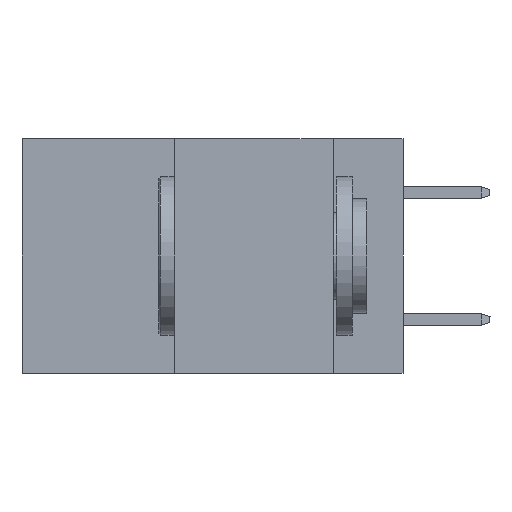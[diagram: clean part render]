
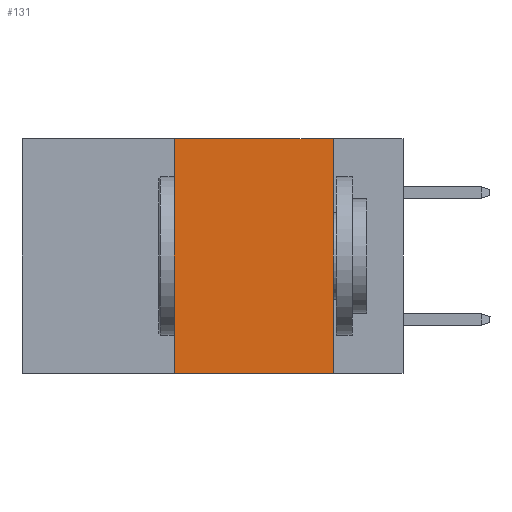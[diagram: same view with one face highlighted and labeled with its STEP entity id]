
A CAD part, left-side view. The second image highlights one B-rep face of the part: STEP entity #131.
In plain terms, the highlighted planar face has unit normal (-1, 0, 0).
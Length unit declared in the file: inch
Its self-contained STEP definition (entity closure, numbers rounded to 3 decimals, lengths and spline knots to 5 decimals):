
#131 = ADVANCED_FACE ( 'NONE', ( #4644 ), #4744, .F. ) ;
#813 = ORIENTED_EDGE ( 'NONE', *, *, #11882, .F. ) ;
#826 = DIRECTION ( 'NONE',  ( 0., -1., 0. ) ) ;
#1549 = LINE ( 'NONE', #8053, #18817 ) ;
#1896 = EDGE_CURVE ( 'NONE', #18761, #7512, #11282, .T. ) ;
#2159 = LINE ( 'NONE', #8363, #12475 ) ;
#2453 = DIRECTION ( 'NONE',  ( 0., 0., 1. ) ) ;
#3088 = ORIENTED_EDGE ( 'NONE', *, *, #19237, .F. ) ;
#3371 = DIRECTION ( 'NONE',  ( 0., 0., -1. ) ) ;
#3776 = ORIENTED_EDGE ( 'NONE', *, *, #13937, .T. ) ;
#4063 = CARTESIAN_POINT ( 'NONE',  ( 0., 0.6, 0. ) ) ;
#4644 = FACE_OUTER_BOUND ( 'NONE', #6862, .T. ) ;
#4744 = PLANE ( 'NONE',  #14690 ) ;
#6140 = CARTESIAN_POINT ( 'NONE',  ( 0., 0.36, -0.37 ) ) ;
#6268 = DIRECTION ( 'NONE',  ( 1., 0., 0. ) ) ;
#6569 = CARTESIAN_POINT ( 'NONE',  ( 0., 0.11, -0.37 ) ) ;
#6862 = EDGE_LOOP ( 'NONE', ( #16992, #3088, #813, #3776 ) ) ;
#7512 = VERTEX_POINT ( 'NONE', #6569 ) ;
#8053 = CARTESIAN_POINT ( 'NONE',  ( 0., 0.6, -0.37 ) ) ;
#8249 = CARTESIAN_POINT ( 'NONE',  ( 0., 0.36, 0. ) ) ;
#8363 = CARTESIAN_POINT ( 'NONE',  ( 0., 0.36, 0. ) ) ;
#9685 = CARTESIAN_POINT ( 'NONE',  ( 0., 0.11, 0. ) ) ;
#11282 = LINE ( 'NONE', #9685, #11466 ) ;
#11466 = VECTOR ( 'NONE', #3371, 39.37008 ) ;
#11876 = VECTOR ( 'NONE', #826, 39.37008 ) ;
#11882 = EDGE_CURVE ( 'NONE', #19713, #19044, #2159, .T. ) ;
#12475 = VECTOR ( 'NONE', #2453, 39.37008 ) ;
#13937 = EDGE_CURVE ( 'NONE', #19713, #7512, #1549, .T. ) ;
#14690 = AXIS2_PLACEMENT_3D ( 'NONE', #18756, #6268, #17122 ) ;
#16992 = ORIENTED_EDGE ( 'NONE', *, *, #1896, .F. ) ;
#17122 = DIRECTION ( 'NONE',  ( 0., 0., -1. ) ) ;
#18756 = CARTESIAN_POINT ( 'NONE',  ( 0., 0.6, 0. ) ) ;
#18761 = VERTEX_POINT ( 'NONE', #19847 ) ;
#18817 = VECTOR ( 'NONE', #20053, 39.37008 ) ;
#19044 = VERTEX_POINT ( 'NONE', #8249 ) ;
#19237 = EDGE_CURVE ( 'NONE', #19044, #18761, #19730, .T. ) ;
#19713 = VERTEX_POINT ( 'NONE', #6140 ) ;
#19730 = LINE ( 'NONE', #4063, #11876 ) ;
#19847 = CARTESIAN_POINT ( 'NONE',  ( 0., 0.11, 0. ) ) ;
#20053 = DIRECTION ( 'NONE',  ( 0., -1., 0. ) ) ;
